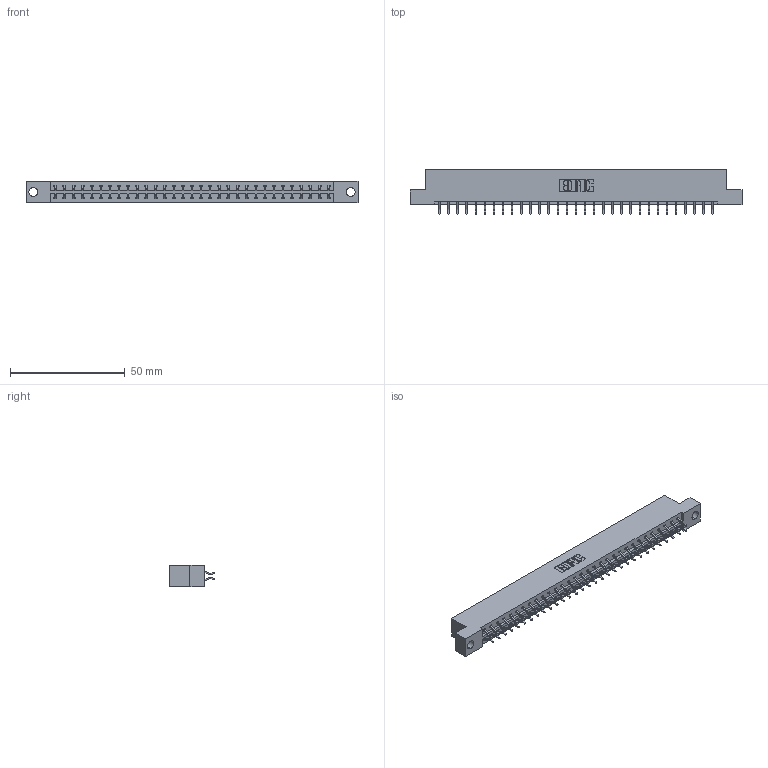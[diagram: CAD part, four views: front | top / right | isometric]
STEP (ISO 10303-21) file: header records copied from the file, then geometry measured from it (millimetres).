
FILE_DESCRIPTION (( 'STEP AP203' ), '1' );
FILE_NAME ('833-062-556-204.STEP', '2020-06-05T06:07:35', ( '' ), ( '' ), 'SwSTEP 2.0', 'SolidWorks 2020', '' );
FILE_SCHEMA (( 'CONFIG_CONTROL_DESIGN' ));
Length unit declared in the file: inch
Products named in the file (3): 833-062-556-204; 833 Part_Flush - .156 Dia - TH; 345-292-001_556 Tail
Assembly tree (63 placements, depth 2):
  833-062-556-204
    833 Part_Flush - .156 Dia - TH
    345-292-001_556 Tail  x62
Bounding box: 144.37 x 19.57 x 9.4 mm (x, y, z)
Volume: 14546.5 mm3; surface area: 16817.7 mm2
Topology: 63 solids, 63 shells, 3710 faces, 11037 edges, 7274 vertices
Faces by surface type: plane 2550, cylinder 1160
Entity records: 21589 total; most frequent: CARTESIAN_POINT 3606, ORIENTED_EDGE 3530, DIRECTION 3089, EDGE_CURVE 1765, LINE 1629, VECTOR 1629, VERTEX_POINT 1174, AXIS2_PLACEMENT_3D 730
